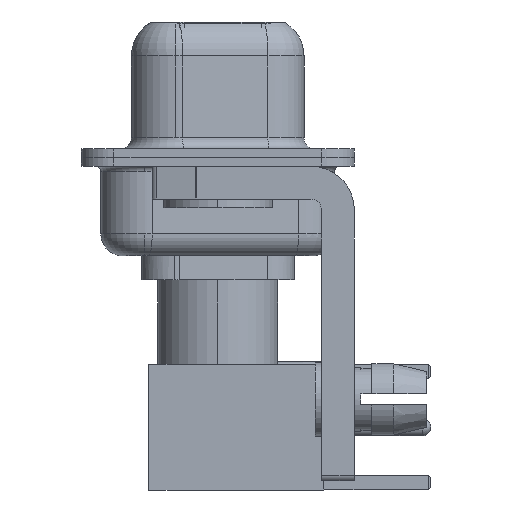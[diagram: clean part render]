
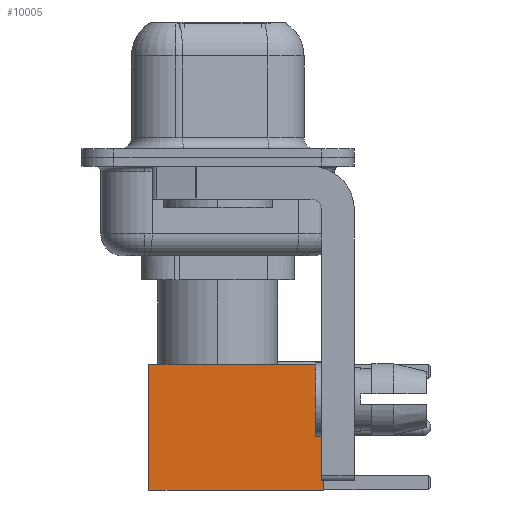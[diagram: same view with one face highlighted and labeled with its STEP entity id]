
A CAD part, left-side view. The second image highlights one B-rep face of the part: STEP entity #10005.
In plain terms, the highlighted face is planar.
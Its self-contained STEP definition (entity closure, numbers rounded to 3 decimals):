
#101 = VERTEX_POINT ( 'NONE', #15711 ) ;
#2656 = VECTOR ( 'NONE', #17286, 1000. ) ;
#2690 = ORIENTED_EDGE ( 'NONE', *, *, #14287, .F. ) ;
#2742 = LINE ( 'NONE', #11006, #2656 ) ;
#3884 = VERTEX_POINT ( 'NONE', #21635 ) ;
#4738 = EDGE_CURVE ( 'NONE', #6396, #3884, #2742, .T. ) ;
#5647 = CARTESIAN_POINT ( 'NONE',  ( 2.875, 2.875, 0. ) ) ;
#6396 = VERTEX_POINT ( 'NONE', #18484 ) ;
#6715 = ORIENTED_EDGE ( 'NONE', *, *, #8017, .T. ) ;
#7571 = VECTOR ( 'NONE', #13818, 1000. ) ;
#7595 = CARTESIAN_POINT ( 'NONE',  ( 0., 2.875, 8. ) ) ;
#7996 = CARTESIAN_POINT ( 'NONE',  ( 2.875, 2.875, 0. ) ) ;
#8017 = EDGE_CURVE ( 'NONE', #101, #23486, #16233, .T. ) ;
#8169 = ORIENTED_EDGE ( 'NONE', *, *, #4738, .F. ) ;
#9492 = CARTESIAN_POINT ( 'NONE',  ( 0., 2.875, 0. ) ) ;
#9556 = CARTESIAN_POINT ( 'NONE',  ( 2.875, 2.875, 0. ) ) ;
#10005 = ADVANCED_FACE ( 'NONE', ( #18370 ), #24405, .T. ) ;
#10594 = VECTOR ( 'NONE', #11597, 1000. ) ;
#10707 = ORIENTED_EDGE ( 'NONE', *, *, #23335, .T. ) ;
#11006 = CARTESIAN_POINT ( 'NONE',  ( -2.875, 2.875, 0. ) ) ;
#11597 = DIRECTION ( 'NONE',  ( 0., 0., -1. ) ) ;
#13818 = DIRECTION ( 'NONE',  ( -1., 0., 0. ) ) ;
#14287 = EDGE_CURVE ( 'NONE', #101, #6396, #19831, .T. ) ;
#15033 = VECTOR ( 'NONE', #18178, 1000. ) ;
#15711 = CARTESIAN_POINT ( 'NONE',  ( 2.875, 2.875, 8. ) ) ;
#16233 = LINE ( 'NONE', #5647, #10594 ) ;
#17286 = DIRECTION ( 'NONE',  ( 0., 0., -1. ) ) ;
#18178 = DIRECTION ( 'NONE',  ( -1., 0., 0. ) ) ;
#18370 = FACE_OUTER_BOUND ( 'NONE', #22975, .T. ) ;
#18484 = CARTESIAN_POINT ( 'NONE',  ( -2.875, 2.875, 8. ) ) ;
#19245 = AXIS2_PLACEMENT_3D ( 'NONE', #9556, #20177, #20306 ) ;
#19831 = LINE ( 'NONE', #7595, #15033 ) ;
#20177 = DIRECTION ( 'NONE',  ( 0., 1., 0. ) ) ;
#20239 = LINE ( 'NONE', #9492, #7571 ) ;
#20306 = DIRECTION ( 'NONE',  ( 0., 0., 1. ) ) ;
#21635 = CARTESIAN_POINT ( 'NONE',  ( -2.875, 2.875, 0. ) ) ;
#22975 = EDGE_LOOP ( 'NONE', ( #6715, #10707, #8169, #2690 ) ) ;
#23335 = EDGE_CURVE ( 'NONE', #23486, #3884, #20239, .T. ) ;
#23486 = VERTEX_POINT ( 'NONE', #7996 ) ;
#24405 = PLANE ( 'NONE',  #19245 ) ;
